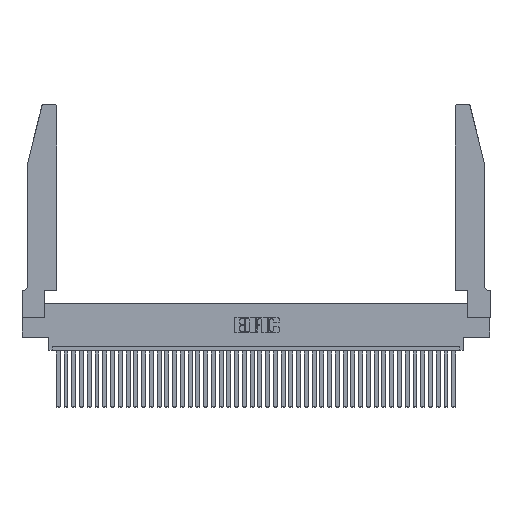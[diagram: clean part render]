
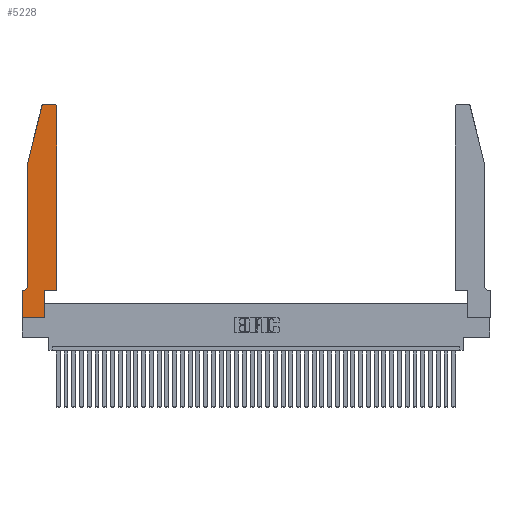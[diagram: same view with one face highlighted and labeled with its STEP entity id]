
A CAD part, top view. The second image highlights one B-rep face of the part: STEP entity #5228.
In plain terms, the highlighted planar face has unit normal (0, 0, 1).
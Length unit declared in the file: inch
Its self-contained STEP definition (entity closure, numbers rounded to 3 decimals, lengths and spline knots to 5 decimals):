
#743 = EDGE_LOOP ( 'NONE', ( #22188, #17522, #10618, #13859, #23391, #16436, #9668, #8998, #18747, #21931, #29178, #37228 ) ) ;
#793 = EDGE_CURVE ( 'NONE', #17103, #1236, #11895, .T. ) ;
#1236 = VERTEX_POINT ( 'NONE', #27796 ) ;
#1532 = LINE ( 'NONE', #4590, #4609 ) ;
#1783 = AXIS2_PLACEMENT_3D ( 'NONE', #2713, #35962, #31599 ) ;
#1888 = VERTEX_POINT ( 'NONE', #14061 ) ;
#2130 = LINE ( 'NONE', #25049, #21610 ) ;
#2239 = CIRCLE ( 'NONE', #26375, 0.07 ) ;
#2713 = CARTESIAN_POINT ( 'NONE',  ( 0.4205, 2.72, 0.37 ) ) ;
#4590 = CARTESIAN_POINT ( 'NONE',  ( 0., 0., 0.37 ) ) ;
#4609 = VECTOR ( 'NONE', #40453, 39.37008 ) ;
#4833 = EDGE_CURVE ( 'NONE', #16772, #35301, #30975, .T. ) ;
#5228 = ADVANCED_FACE ( 'NONE', ( #14503 ), #31270, .T. ) ;
#5384 = DIRECTION ( 'NONE',  ( 0., 0., 1. ) ) ;
#5661 = DIRECTION ( 'NONE',  ( 1., 0., 0. ) ) ;
#6636 = EDGE_CURVE ( 'NONE', #29882, #16772, #2130, .T. ) ;
#6999 = EDGE_CURVE ( 'NONE', #1236, #32222, #1532, .T. ) ;
#7906 = CARTESIAN_POINT ( 'NONE',  ( 0.2865, 0.35, 0.37 ) ) ;
#8421 = DIRECTION ( 'NONE',  ( 1., 0., 0. ) ) ;
#8829 = CARTESIAN_POINT ( 'NONE',  ( 0., 0.35, 0.37 ) ) ;
#8998 = ORIENTED_EDGE ( 'NONE', *, *, #24229, .T. ) ;
#9338 = VERTEX_POINT ( 'NONE', #14348 ) ;
#9668 = ORIENTED_EDGE ( 'NONE', *, *, #6999, .T. ) ;
#9732 = LINE ( 'NONE', #12179, #31744 ) ;
#9882 = VECTOR ( 'NONE', #38191, 39.37008 ) ;
#9969 = VERTEX_POINT ( 'NONE', #21348 ) ;
#10445 = CARTESIAN_POINT ( 'NONE',  ( 0.0755, 0.42, 0.37 ) ) ;
#10618 = ORIENTED_EDGE ( 'NONE', *, *, #40822, .T. ) ;
#11241 = CARTESIAN_POINT ( 'NONE',  ( 0.284, 2.72, 0.37 ) ) ;
#11550 = LINE ( 'NONE', #27016, #27456 ) ;
#11851 = VECTOR ( 'NONE', #28833, 39.37008 ) ;
#11895 = LINE ( 'NONE', #25859, #11851 ) ;
#12179 = CARTESIAN_POINT ( 'NONE',  ( 0.0755, 2., 0.37 ) ) ;
#12537 = EDGE_CURVE ( 'NONE', #35301, #9969, #21708, .T. ) ;
#13859 = ORIENTED_EDGE ( 'NONE', *, *, #25695, .T. ) ;
#14061 = CARTESIAN_POINT ( 'NONE',  ( 0.0755, 2., 0.37 ) ) ;
#14348 = CARTESIAN_POINT ( 'NONE',  ( 0.284, 2.75, 0.37 ) ) ;
#14503 = FACE_OUTER_BOUND ( 'NONE', #743, .T. ) ;
#14657 = DIRECTION ( 'NONE',  ( 0., 0., 1. ) ) ;
#14800 = CIRCLE ( 'NONE', #25853, 0.03 ) ;
#15115 = AXIS2_PLACEMENT_3D ( 'NONE', #8829, #5384, #5661 ) ;
#15750 = DIRECTION ( 'NONE',  ( -1., 0., 0. ) ) ;
#16436 = ORIENTED_EDGE ( 'NONE', *, *, #793, .T. ) ;
#16578 = VECTOR ( 'NONE', #38351, 39.37008 ) ;
#16772 = VERTEX_POINT ( 'NONE', #39985 ) ;
#17103 = VERTEX_POINT ( 'NONE', #31374 ) ;
#17296 = CARTESIAN_POINT ( 'NONE',  ( 0.2605, 2.75, 0.37 ) ) ;
#17522 = ORIENTED_EDGE ( 'NONE', *, *, #17838, .T. ) ;
#17838 = EDGE_CURVE ( 'NONE', #9338, #24950, #14800, .T. ) ;
#18417 = LINE ( 'NONE', #17296, #21513 ) ;
#18747 = ORIENTED_EDGE ( 'NONE', *, *, #24301, .T. ) ;
#20120 = VECTOR ( 'NONE', #21694, 39.37008 ) ;
#20411 = DIRECTION ( 'NONE',  ( -0.239, -0.971, 0. ) ) ;
#21348 = CARTESIAN_POINT ( 'NONE',  ( 0.4205, 2.75, 0.37 ) ) ;
#21513 = VECTOR ( 'NONE', #30513, 39.37008 ) ;
#21610 = VECTOR ( 'NONE', #8421, 39.37008 ) ;
#21694 = DIRECTION ( 'NONE',  ( 0., 1., 0. ) ) ;
#21708 = CIRCLE ( 'NONE', #1783, 0.03 ) ;
#21931 = ORIENTED_EDGE ( 'NONE', *, *, #6636, .T. ) ;
#21934 = CARTESIAN_POINT ( 'NONE',  ( 0.25487, 2.72718, 0.37 ) ) ;
#22188 = ORIENTED_EDGE ( 'NONE', *, *, #25912, .T. ) ;
#22476 = CARTESIAN_POINT ( 'NONE',  ( 0.4505, 2.72, 0.37 ) ) ;
#22584 = CARTESIAN_POINT ( 'NONE',  ( 0.4505, 0.35, 0.37 ) ) ;
#23094 = CARTESIAN_POINT ( 'NONE',  ( 0., 0., 0.37 ) ) ;
#23391 = ORIENTED_EDGE ( 'NONE', *, *, #41843, .T. ) ;
#24229 = EDGE_CURVE ( 'NONE', #32222, #36181, #28834, .T. ) ;
#24301 = EDGE_CURVE ( 'NONE', #36181, #29882, #33966, .T. ) ;
#24950 = VERTEX_POINT ( 'NONE', #21934 ) ;
#25049 = CARTESIAN_POINT ( 'NONE',  ( 0.4505, 0.35, 0.37 ) ) ;
#25311 = DIRECTION ( 'NONE',  ( 1., 0., 0. ) ) ;
#25695 = EDGE_CURVE ( 'NONE', #1888, #35723, #9732, .T. ) ;
#25853 = AXIS2_PLACEMENT_3D ( 'NONE', #11241, #14657, #25311 ) ;
#25859 = CARTESIAN_POINT ( 'NONE',  ( 0.0755, 0.35, 0.37 ) ) ;
#25912 = EDGE_CURVE ( 'NONE', #9969, #9338, #18417, .T. ) ;
#26375 = AXIS2_PLACEMENT_3D ( 'NONE', #35852, #39150, #15750 ) ;
#27016 = CARTESIAN_POINT ( 'NONE',  ( 0.0755, 2., 0.37 ) ) ;
#27456 = VECTOR ( 'NONE', #20411, 39.37008 ) ;
#27796 = CARTESIAN_POINT ( 'NONE',  ( 0., 0.35, 0.37 ) ) ;
#28570 = CARTESIAN_POINT ( 'NONE',  ( 0.2865, 0.35, 0.37 ) ) ;
#28833 = DIRECTION ( 'NONE',  ( -1., 0., 0. ) ) ;
#28834 = LINE ( 'NONE', #31422, #9882 ) ;
#29178 = ORIENTED_EDGE ( 'NONE', *, *, #4833, .T. ) ;
#29882 = VERTEX_POINT ( 'NONE', #7906 ) ;
#30317 = CARTESIAN_POINT ( 'NONE',  ( 0.2865, 0., 0.37 ) ) ;
#30513 = DIRECTION ( 'NONE',  ( -1., 0., 0. ) ) ;
#30975 = LINE ( 'NONE', #22584, #16578 ) ;
#31270 = PLANE ( 'NONE',  #15115 ) ;
#31374 = CARTESIAN_POINT ( 'NONE',  ( 0.0055, 0.35, 0.37 ) ) ;
#31422 = CARTESIAN_POINT ( 'NONE',  ( 0., 0., 0.37 ) ) ;
#31599 = DIRECTION ( 'NONE',  ( 1., 0., 0. ) ) ;
#31744 = VECTOR ( 'NONE', #32086, 39.37008 ) ;
#32086 = DIRECTION ( 'NONE',  ( 0., -1., 0. ) ) ;
#32222 = VERTEX_POINT ( 'NONE', #23094 ) ;
#33966 = LINE ( 'NONE', #28570, #20120 ) ;
#35301 = VERTEX_POINT ( 'NONE', #22476 ) ;
#35723 = VERTEX_POINT ( 'NONE', #10445 ) ;
#35852 = CARTESIAN_POINT ( 'NONE',  ( 0.0055, 0.42, 0.37 ) ) ;
#35962 = DIRECTION ( 'NONE',  ( 0., 0., 1. ) ) ;
#36181 = VERTEX_POINT ( 'NONE', #30317 ) ;
#37228 = ORIENTED_EDGE ( 'NONE', *, *, #12537, .T. ) ;
#38191 = DIRECTION ( 'NONE',  ( 1., 0., 0. ) ) ;
#38351 = DIRECTION ( 'NONE',  ( 0., 1., 0. ) ) ;
#39150 = DIRECTION ( 'NONE',  ( 0., 0., -1. ) ) ;
#39985 = CARTESIAN_POINT ( 'NONE',  ( 0.4505, 0.35, 0.37 ) ) ;
#40453 = DIRECTION ( 'NONE',  ( 0., -1., 0. ) ) ;
#40822 = EDGE_CURVE ( 'NONE', #24950, #1888, #11550, .T. ) ;
#41843 = EDGE_CURVE ( 'NONE', #35723, #17103, #2239, .T. ) ;
